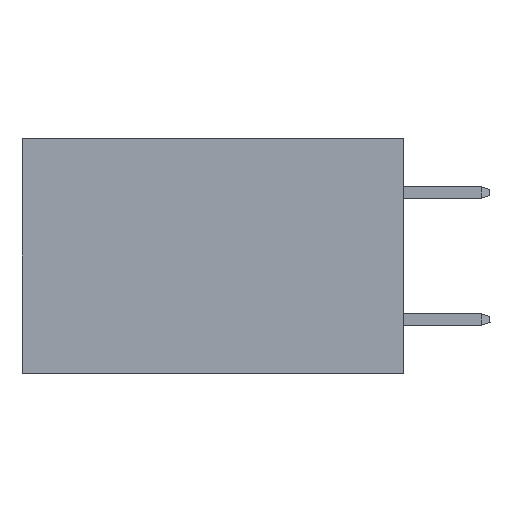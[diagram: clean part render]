
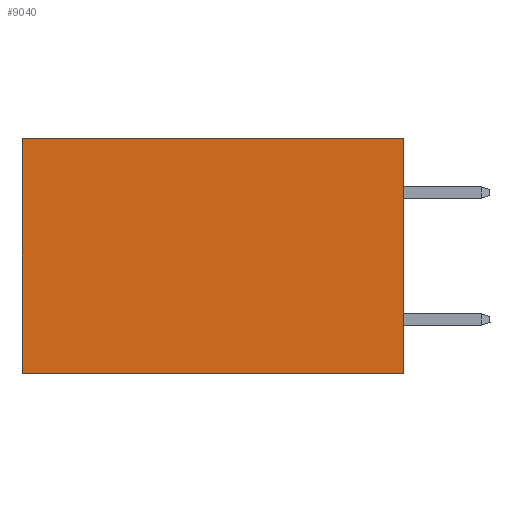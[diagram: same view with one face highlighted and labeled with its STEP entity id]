
A CAD part, left-side view. The second image highlights one B-rep face of the part: STEP entity #9040.
In plain terms, the highlighted planar face has unit normal (-1, 0, 0).
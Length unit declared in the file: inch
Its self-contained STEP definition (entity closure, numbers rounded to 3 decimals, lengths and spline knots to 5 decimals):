
#431 = PLANE ( 'NONE',  #1508 ) ;
#1335 = CARTESIAN_POINT ( 'NONE',  ( 0.2875, 0.6, 0. ) ) ;
#1392 = CARTESIAN_POINT ( 'NONE',  ( 0.2875, 0.6, 0. ) ) ;
#1508 = AXIS2_PLACEMENT_3D ( 'NONE', #15421, #5178, #24257 ) ;
#3033 = VECTOR ( 'NONE', #13351, 39.37008 ) ;
#4361 = CARTESIAN_POINT ( 'NONE',  ( 0.2875, 0., -0.37 ) ) ;
#5032 = CARTESIAN_POINT ( 'NONE',  ( 0.2875, 0., 0. ) ) ;
#5178 = DIRECTION ( 'NONE',  ( 1., 0., 0. ) ) ;
#5342 = ORIENTED_EDGE ( 'NONE', *, *, #21144, .T. ) ;
#5400 = EDGE_CURVE ( 'NONE', #10110, #11475, #5838, .T. ) ;
#5838 = LINE ( 'NONE', #22457, #3033 ) ;
#6383 = VERTEX_POINT ( 'NONE', #1335 ) ;
#6703 = LINE ( 'NONE', #1392, #19912 ) ;
#6876 = CARTESIAN_POINT ( 'NONE',  ( 0.2875, 0., 0. ) ) ;
#8685 = DIRECTION ( 'NONE',  ( 0., 0., -1. ) ) ;
#9040 = ADVANCED_FACE ( 'NONE', ( #16240 ), #431, .F. ) ;
#9484 = ORIENTED_EDGE ( 'NONE', *, *, #5400, .F. ) ;
#10110 = VERTEX_POINT ( 'NONE', #6876 ) ;
#11301 = EDGE_CURVE ( 'NONE', #11475, #21202, #15530, .T. ) ;
#11475 = VERTEX_POINT ( 'NONE', #16618 ) ;
#11585 = ORIENTED_EDGE ( 'NONE', *, *, #16098, .T. ) ;
#11870 = DIRECTION ( 'NONE',  ( 0., 1., 0. ) ) ;
#13351 = DIRECTION ( 'NONE',  ( 0., 0., -1. ) ) ;
#15421 = CARTESIAN_POINT ( 'NONE',  ( 0.2875, 0., 0. ) ) ;
#15530 = LINE ( 'NONE', #4361, #20784 ) ;
#16093 = LINE ( 'NONE', #5032, #23201 ) ;
#16098 = EDGE_CURVE ( 'NONE', #6383, #21202, #6703, .T. ) ;
#16240 = FACE_OUTER_BOUND ( 'NONE', #22262, .T. ) ;
#16618 = CARTESIAN_POINT ( 'NONE',  ( 0.2875, 0., -0.37 ) ) ;
#17111 = ORIENTED_EDGE ( 'NONE', *, *, #11301, .F. ) ;
#17184 = CARTESIAN_POINT ( 'NONE',  ( 0.2875, 0.6, -0.37 ) ) ;
#19912 = VECTOR ( 'NONE', #8685, 39.37008 ) ;
#20784 = VECTOR ( 'NONE', #11870, 39.37008 ) ;
#21144 = EDGE_CURVE ( 'NONE', #10110, #6383, #16093, .T. ) ;
#21202 = VERTEX_POINT ( 'NONE', #17184 ) ;
#22262 = EDGE_LOOP ( 'NONE', ( #11585, #17111, #9484, #5342 ) ) ;
#22457 = CARTESIAN_POINT ( 'NONE',  ( 0.2875, 0., 0. ) ) ;
#23201 = VECTOR ( 'NONE', #23411, 39.37008 ) ;
#23411 = DIRECTION ( 'NONE',  ( 0., 1., 0. ) ) ;
#24257 = DIRECTION ( 'NONE',  ( 0., 0., -1. ) ) ;
